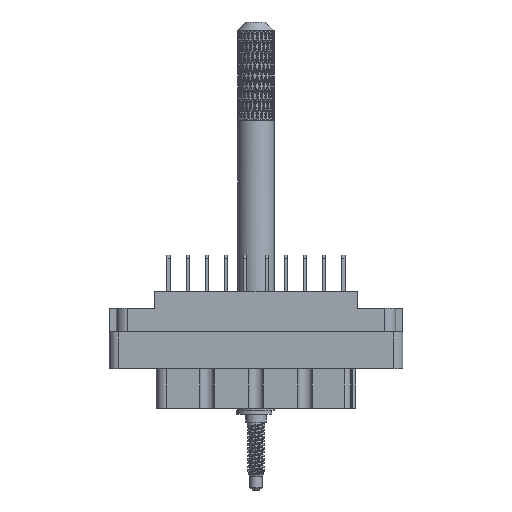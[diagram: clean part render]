
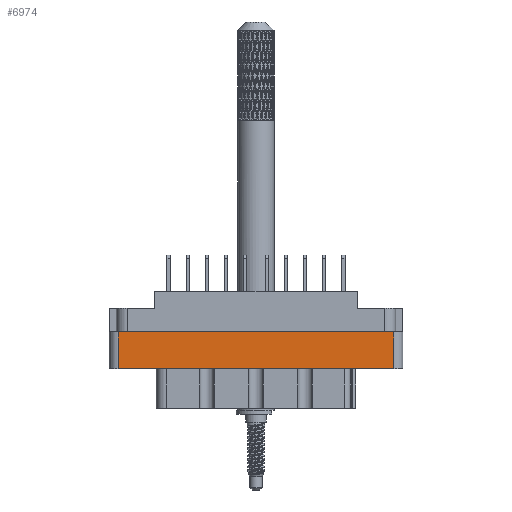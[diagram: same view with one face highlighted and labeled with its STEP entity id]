
A CAD part, front view. The second image highlights one B-rep face of the part: STEP entity #6974.
In plain terms, the highlighted planar face has unit normal (0, -1, 0).
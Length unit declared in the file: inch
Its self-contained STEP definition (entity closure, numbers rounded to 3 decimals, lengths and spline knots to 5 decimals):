
#177 = EDGE_CURVE ( 'NONE', #42102, #43712, #23569, .T. ) ;
#3974 = LINE ( 'NONE', #18139, #25465 ) ;
#6729 = VERTEX_POINT ( 'NONE', #89231 ) ;
#6974 = ADVANCED_FACE ( 'NONE', ( #76802 ), #31567, .T. ) ;
#7877 = DIRECTION ( 'NONE',  ( 0., 0., -1. ) ) ;
#8837 = ORIENTED_EDGE ( 'NONE', *, *, #14279, .F. ) ;
#11220 = CARTESIAN_POINT ( 'NONE',  ( -0.938, -0.438, -0.798 ) ) ;
#14279 = EDGE_CURVE ( 'NONE', #6729, #43712, #3974, .T. ) ;
#15261 = ORIENTED_EDGE ( 'NONE', *, *, #177, .T. ) ;
#18139 = CARTESIAN_POINT ( 'NONE',  ( 0., -0.438, -0.529 ) ) ;
#20849 = VECTOR ( 'NONE', #82931, 39.37008 ) ;
#23569 = LINE ( 'NONE', #11220, #61479 ) ;
#25465 = VECTOR ( 'NONE', #99708, 39.37008 ) ;
#26650 = CARTESIAN_POINT ( 'NONE',  ( -0.938, -0.438, -0.529 ) ) ;
#27779 = VERTEX_POINT ( 'NONE', #81089 ) ;
#28572 = ORIENTED_EDGE ( 'NONE', *, *, #56384, .F. ) ;
#31567 = PLANE ( 'NONE',  #33253 ) ;
#33253 = AXIS2_PLACEMENT_3D ( 'NONE', #96170, #64050, #7877 ) ;
#34543 = CARTESIAN_POINT ( 'NONE',  ( -0.938, -0.438, -0.277 ) ) ;
#42102 = VERTEX_POINT ( 'NONE', #34543 ) ;
#43169 = EDGE_CURVE ( 'NONE', #6729, #27779, #83975, .T. ) ;
#43712 = VERTEX_POINT ( 'NONE', #26650 ) ;
#49280 = EDGE_LOOP ( 'NONE', ( #28572, #15261, #8837, #92367 ) ) ;
#50891 = DIRECTION ( 'NONE',  ( 0., 0., -1. ) ) ;
#56384 = EDGE_CURVE ( 'NONE', #42102, #27779, #64887, .T. ) ;
#61479 = VECTOR ( 'NONE', #50891, 39.37008 ) ;
#64050 = DIRECTION ( 'NONE',  ( 0., -1., 0. ) ) ;
#64887 = LINE ( 'NONE', #82578, #87656 ) ;
#65987 = CARTESIAN_POINT ( 'NONE',  ( 0.938, -0.438, -0.798 ) ) ;
#76802 = FACE_OUTER_BOUND ( 'NONE', #49280, .T. ) ;
#81089 = CARTESIAN_POINT ( 'NONE',  ( 0.938, -0.438, -0.277 ) ) ;
#82578 = CARTESIAN_POINT ( 'NONE',  ( 0., -0.438, -0.277 ) ) ;
#82931 = DIRECTION ( 'NONE',  ( 0., 0., 1. ) ) ;
#83975 = LINE ( 'NONE', #65987, #20849 ) ;
#87656 = VECTOR ( 'NONE', #98475, 39.37008 ) ;
#89231 = CARTESIAN_POINT ( 'NONE',  ( 0.938, -0.438, -0.529 ) ) ;
#92367 = ORIENTED_EDGE ( 'NONE', *, *, #43169, .T. ) ;
#96170 = CARTESIAN_POINT ( 'NONE',  ( -1., -0.438, -0.798 ) ) ;
#98475 = DIRECTION ( 'NONE',  ( 1., 0., 0. ) ) ;
#99708 = DIRECTION ( 'NONE',  ( -1., 0., 0. ) ) ;
